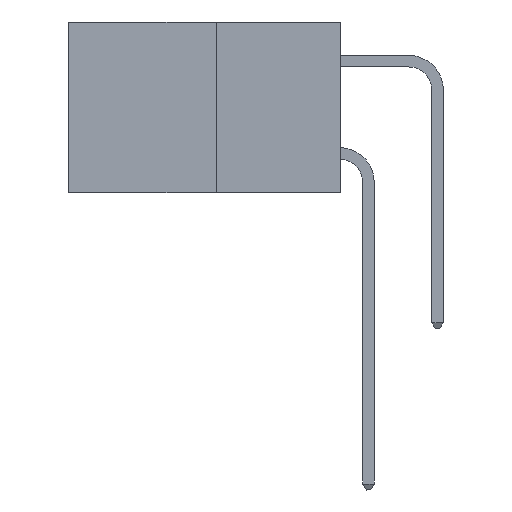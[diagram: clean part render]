
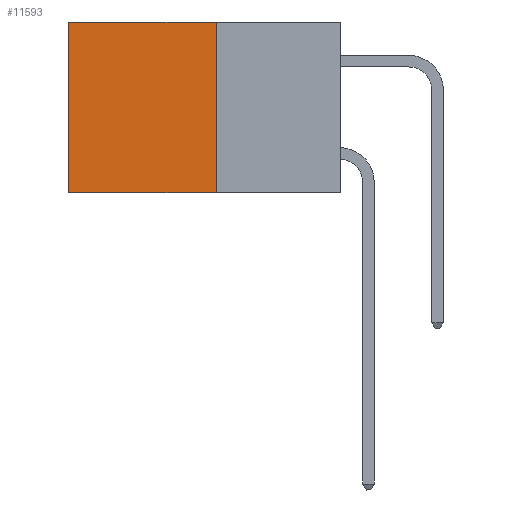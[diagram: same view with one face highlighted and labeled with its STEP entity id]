
A CAD part, left-side view. The second image highlights one B-rep face of the part: STEP entity #11593.
In plain terms, the highlighted planar face has unit normal (-1, 0, 0).
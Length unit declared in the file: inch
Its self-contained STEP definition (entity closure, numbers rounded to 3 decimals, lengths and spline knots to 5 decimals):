
#34 = LINE ( 'NONE', #1331, #10832 ) ;
#607 = CARTESIAN_POINT ( 'NONE',  ( 0.277, 0.59, -0.37 ) ) ;
#725 = CARTESIAN_POINT ( 'NONE',  ( 0.277, 0.27, -0.37 ) ) ;
#922 = FACE_OUTER_BOUND ( 'NONE', #5923, .T. ) ;
#1015 = EDGE_CURVE ( 'NONE', #2380, #4537, #1419, .T. ) ;
#1082 = VECTOR ( 'NONE', #11980, 39.37008 ) ;
#1331 = CARTESIAN_POINT ( 'NONE',  ( 0.277, 0.27, -0.37 ) ) ;
#1419 = LINE ( 'NONE', #5511, #1082 ) ;
#1449 = VECTOR ( 'NONE', #4460, 39.37008 ) ;
#1653 = LINE ( 'NONE', #3196, #6885 ) ;
#2380 = VERTEX_POINT ( 'NONE', #3059 ) ;
#3059 = CARTESIAN_POINT ( 'NONE',  ( 0.277, 0.27, 0. ) ) ;
#3063 = PLANE ( 'NONE',  #12290 ) ;
#3196 = CARTESIAN_POINT ( 'NONE',  ( 0.277, 0.27, 0. ) ) ;
#3437 = CARTESIAN_POINT ( 'NONE',  ( 0.277, 0.59, -0.37 ) ) ;
#4060 = VERTEX_POINT ( 'NONE', #5714 ) ;
#4112 = DIRECTION ( 'NONE',  ( 0., 0., -1. ) ) ;
#4228 = LINE ( 'NONE', #3437, #1449 ) ;
#4460 = DIRECTION ( 'NONE',  ( 0., 0., -1. ) ) ;
#4537 = VERTEX_POINT ( 'NONE', #725 ) ;
#5511 = CARTESIAN_POINT ( 'NONE',  ( 0.277, 0.27, -0.37 ) ) ;
#5672 = VERTEX_POINT ( 'NONE', #607 ) ;
#5714 = CARTESIAN_POINT ( 'NONE',  ( 0.277, 0.59, 0. ) ) ;
#5923 = EDGE_LOOP ( 'NONE', ( #9456, #8050, #6617, #12371 ) ) ;
#6576 = DIRECTION ( 'NONE',  ( 0., 1., 0. ) ) ;
#6617 = ORIENTED_EDGE ( 'NONE', *, *, #1015, .F. ) ;
#6885 = VECTOR ( 'NONE', #12302, 39.37008 ) ;
#7116 = EDGE_CURVE ( 'NONE', #2380, #4060, #1653, .T. ) ;
#7210 = CARTESIAN_POINT ( 'NONE',  ( 0.277, 0.27, -0.37 ) ) ;
#7485 = EDGE_CURVE ( 'NONE', #4537, #5672, #34, .T. ) ;
#8050 = ORIENTED_EDGE ( 'NONE', *, *, #7485, .F. ) ;
#9456 = ORIENTED_EDGE ( 'NONE', *, *, #10634, .T. ) ;
#10273 = DIRECTION ( 'NONE',  ( 1., 0., 0. ) ) ;
#10634 = EDGE_CURVE ( 'NONE', #4060, #5672, #4228, .T. ) ;
#10832 = VECTOR ( 'NONE', #6576, 39.37008 ) ;
#11593 = ADVANCED_FACE ( 'NONE', ( #922 ), #3063, .F. ) ;
#11980 = DIRECTION ( 'NONE',  ( 0., 0., -1. ) ) ;
#12290 = AXIS2_PLACEMENT_3D ( 'NONE', #7210, #10273, #4112 ) ;
#12302 = DIRECTION ( 'NONE',  ( 0., 1., 0. ) ) ;
#12371 = ORIENTED_EDGE ( 'NONE', *, *, #7116, .T. ) ;
